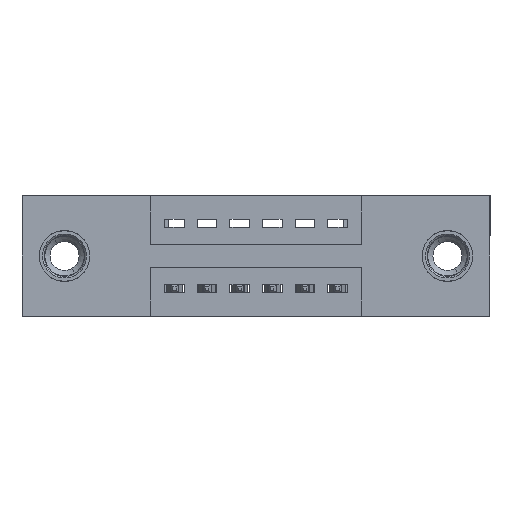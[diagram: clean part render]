
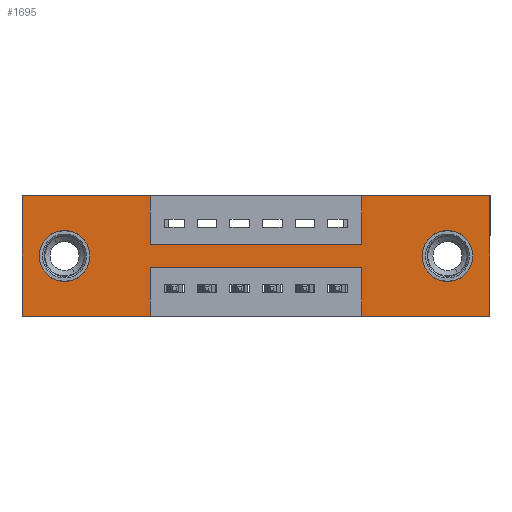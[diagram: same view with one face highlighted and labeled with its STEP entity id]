
A CAD part, front view. The second image highlights one B-rep face of the part: STEP entity #1695.
In plain terms, the highlighted planar face has unit normal (0, -1, 0).
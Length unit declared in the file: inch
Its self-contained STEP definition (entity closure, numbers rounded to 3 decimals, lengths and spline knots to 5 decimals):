
#74 = VECTOR ( 'NONE', #6606, 39.37008 ) ;
#309 = AXIS2_PLACEMENT_3D ( 'NONE', #6542, #10901, #5456 ) ;
#311 = FACE_OUTER_BOUND ( 'NONE', #3022, .T. ) ;
#397 = LINE ( 'NONE', #5510, #74 ) ;
#507 = VERTEX_POINT ( 'NONE', #11267 ) ;
#518 = CARTESIAN_POINT ( 'NONE',  ( 1.0425, 0., -0.22 ) ) ;
#690 = CIRCLE ( 'NONE', #8399, 0.078 ) ;
#788 = VERTEX_POINT ( 'NONE', #11175 ) ;
#956 = VERTEX_POINT ( 'NONE', #5908 ) ;
#1000 = VERTEX_POINT ( 'NONE', #10534 ) ;
#1104 = AXIS2_PLACEMENT_3D ( 'NONE', #5994, #8151, #4894 ) ;
#1392 = EDGE_CURVE ( 'NONE', #956, #8278, #1868, .T. ) ;
#1492 = ORIENTED_EDGE ( 'NONE', *, *, #8976, .F. ) ;
#1536 = ORIENTED_EDGE ( 'NONE', *, *, #10823, .T. ) ;
#1582 = CARTESIAN_POINT ( 'NONE',  ( 0., 0., -0.37 ) ) ;
#1606 = LINE ( 'NONE', #8634, #13543 ) ;
#1695 = ADVANCED_FACE ( 'NONE', ( #12281, #9045, #311 ), #2834, .T. ) ;
#1771 = DIRECTION ( 'NONE',  ( -1., 0., 0. ) ) ;
#1868 = CIRCLE ( 'NONE', #9289, 0.078 ) ;
#1903 = VERTEX_POINT ( 'NONE', #7016 ) ;
#1915 = CARTESIAN_POINT ( 'NONE',  ( 1.0425, 0., -0.37 ) ) ;
#1928 = ORIENTED_EDGE ( 'NONE', *, *, #3290, .F. ) ;
#2339 = VECTOR ( 'NONE', #7646, 39.37008 ) ;
#2377 = DIRECTION ( 'NONE',  ( 1., 0., 0. ) ) ;
#2423 = VERTEX_POINT ( 'NONE', #12396 ) ;
#2514 = EDGE_CURVE ( 'NONE', #3822, #8650, #5929, .T. ) ;
#2618 = ORIENTED_EDGE ( 'NONE', *, *, #8260, .F. ) ;
#2637 = ORIENTED_EDGE ( 'NONE', *, *, #5475, .F. ) ;
#2798 = AXIS2_PLACEMENT_3D ( 'NONE', #13715, #9388, #8246 ) ;
#2834 = PLANE ( 'NONE',  #2798 ) ;
#2943 = DIRECTION ( 'NONE',  ( 0., 0., 1. ) ) ;
#3022 = EDGE_LOOP ( 'NONE', ( #2618, #10832, #9074, #12781, #4828, #5292, #6846, #13736, #1928, #1492, #11619, #2637 ) ) ;
#3081 = CARTESIAN_POINT ( 'NONE',  ( 0.3925, 0., -0.15 ) ) ;
#3090 = LINE ( 'NONE', #3841, #5827 ) ;
#3159 = DIRECTION ( 'NONE',  ( 0., 0., 1. ) ) ;
#3215 = EDGE_CURVE ( 'NONE', #788, #1000, #3816, .T. ) ;
#3290 = EDGE_CURVE ( 'NONE', #1903, #788, #1606, .T. ) ;
#3531 = LINE ( 'NONE', #7357, #7301 ) ;
#3583 = VECTOR ( 'NONE', #1771, 39.37008 ) ;
#3816 = LINE ( 'NONE', #3081, #12546 ) ;
#3822 = VERTEX_POINT ( 'NONE', #10755 ) ;
#3833 = VECTOR ( 'NONE', #6990, 39.37008 ) ;
#3841 = CARTESIAN_POINT ( 'NONE',  ( 0., 0., -0.37 ) ) ;
#4026 = CARTESIAN_POINT ( 'NONE',  ( 1.305, 0., -0.107 ) ) ;
#4513 = DIRECTION ( 'NONE',  ( 0., 0., -1. ) ) ;
#4688 = CARTESIAN_POINT ( 'NONE',  ( 0., 0., 0. ) ) ;
#4800 = CARTESIAN_POINT ( 'NONE',  ( 0.3925, 0., -0.22 ) ) ;
#4828 = ORIENTED_EDGE ( 'NONE', *, *, #9532, .F. ) ;
#4894 = DIRECTION ( 'NONE',  ( 0., 0., -1. ) ) ;
#4933 = ORIENTED_EDGE ( 'NONE', *, *, #14075, .T. ) ;
#5292 = ORIENTED_EDGE ( 'NONE', *, *, #12111, .F. ) ;
#5301 = LINE ( 'NONE', #1582, #3583 ) ;
#5400 = CIRCLE ( 'NONE', #1104, 0.078 ) ;
#5426 = DIRECTION ( 'NONE',  ( 0., 0., 1. ) ) ;
#5456 = DIRECTION ( 'NONE',  ( 0., 0., 1. ) ) ;
#5467 = DIRECTION ( 'NONE',  ( 0., 1., 0. ) ) ;
#5475 = EDGE_CURVE ( 'NONE', #10353, #507, #5301, .T. ) ;
#5510 = CARTESIAN_POINT ( 'NONE',  ( 0., 0., 0. ) ) ;
#5827 = VECTOR ( 'NONE', #13760, 39.37008 ) ;
#5908 = CARTESIAN_POINT ( 'NONE',  ( 0.13, 0., -0.107 ) ) ;
#5929 = LINE ( 'NONE', #1915, #9528 ) ;
#5994 = CARTESIAN_POINT ( 'NONE',  ( 1.305, 0., -0.185 ) ) ;
#6279 = DIRECTION ( 'NONE',  ( 1., 0., 0. ) ) ;
#6542 = CARTESIAN_POINT ( 'NONE',  ( 0.13, 0., -0.185 ) ) ;
#6561 = CARTESIAN_POINT ( 'NONE',  ( 0.13, 0., -0.185 ) ) ;
#6584 = CARTESIAN_POINT ( 'NONE',  ( 0.3925, 0., -0.37 ) ) ;
#6606 = DIRECTION ( 'NONE',  ( 1., 0., 0. ) ) ;
#6846 = ORIENTED_EDGE ( 'NONE', *, *, #7122, .F. ) ;
#6886 = VERTEX_POINT ( 'NONE', #7288 ) ;
#6990 = DIRECTION ( 'NONE',  ( -1., 0., 0. ) ) ;
#7016 = CARTESIAN_POINT ( 'NONE',  ( 0.3925, 0., 0. ) ) ;
#7122 = EDGE_CURVE ( 'NONE', #1000, #12155, #3531, .T. ) ;
#7231 = EDGE_LOOP ( 'NONE', ( #8929, #4933 ) ) ;
#7288 = CARTESIAN_POINT ( 'NONE',  ( 1.435, 0., 0. ) ) ;
#7301 = VECTOR ( 'NONE', #3159, 39.37008 ) ;
#7357 = CARTESIAN_POINT ( 'NONE',  ( 1.0425, 0., 0. ) ) ;
#7638 = LINE ( 'NONE', #6584, #2339 ) ;
#7646 = DIRECTION ( 'NONE',  ( 0., 0., -1. ) ) ;
#7792 = LINE ( 'NONE', #8923, #13579 ) ;
#7817 = CARTESIAN_POINT ( 'NONE',  ( 0.3925, 0., -0.37 ) ) ;
#7849 = VERTEX_POINT ( 'NONE', #11430 ) ;
#7851 = CARTESIAN_POINT ( 'NONE',  ( 1.305, 0., -0.185 ) ) ;
#7939 = DIRECTION ( 'NONE',  ( 0., 1., 0. ) ) ;
#7961 = EDGE_CURVE ( 'NONE', #9775, #2423, #5400, .T. ) ;
#8151 = DIRECTION ( 'NONE',  ( 0., 1., 0. ) ) ;
#8246 = DIRECTION ( 'NONE',  ( 0., 0., -1. ) ) ;
#8260 = EDGE_CURVE ( 'NONE', #13501, #10353, #7638, .T. ) ;
#8278 = VERTEX_POINT ( 'NONE', #10941 ) ;
#8399 = AXIS2_PLACEMENT_3D ( 'NONE', #7851, #7939, #4513 ) ;
#8630 = LINE ( 'NONE', #11278, #12056 ) ;
#8634 = CARTESIAN_POINT ( 'NONE',  ( 0.3925, 0., 0. ) ) ;
#8650 = VERTEX_POINT ( 'NONE', #518 ) ;
#8923 = CARTESIAN_POINT ( 'NONE',  ( 0., 0., 0. ) ) ;
#8929 = ORIENTED_EDGE ( 'NONE', *, *, #7961, .T. ) ;
#8959 = ORIENTED_EDGE ( 'NONE', *, *, #1392, .T. ) ;
#8976 = EDGE_CURVE ( 'NONE', #7849, #1903, #7792, .T. ) ;
#9045 = FACE_BOUND ( 'NONE', #11641, .T. ) ;
#9054 = DIRECTION ( 'NONE',  ( 0., 0., -1. ) ) ;
#9074 = ORIENTED_EDGE ( 'NONE', *, *, #2514, .F. ) ;
#9289 = AXIS2_PLACEMENT_3D ( 'NONE', #6561, #5467, #5426 ) ;
#9388 = DIRECTION ( 'NONE',  ( 0., -1., 0. ) ) ;
#9508 = EDGE_CURVE ( 'NONE', #8650, #13501, #11539, .T. ) ;
#9528 = VECTOR ( 'NONE', #9552, 39.37008 ) ;
#9532 = EDGE_CURVE ( 'NONE', #6886, #10558, #8630, .T. ) ;
#9552 = DIRECTION ( 'NONE',  ( 0., 0., 1. ) ) ;
#9775 = VERTEX_POINT ( 'NONE', #4026 ) ;
#9892 = LINE ( 'NONE', #4688, #12656 ) ;
#10007 = CIRCLE ( 'NONE', #309, 0.078 ) ;
#10031 = EDGE_CURVE ( 'NONE', #507, #7849, #9892, .T. ) ;
#10353 = VERTEX_POINT ( 'NONE', #7817 ) ;
#10534 = CARTESIAN_POINT ( 'NONE',  ( 1.0425, 0., -0.15 ) ) ;
#10558 = VERTEX_POINT ( 'NONE', #12588 ) ;
#10755 = CARTESIAN_POINT ( 'NONE',  ( 1.0425, 0., -0.37 ) ) ;
#10823 = EDGE_CURVE ( 'NONE', #8278, #956, #10007, .T. ) ;
#10832 = ORIENTED_EDGE ( 'NONE', *, *, #9508, .F. ) ;
#10901 = DIRECTION ( 'NONE',  ( 0., 1., 0. ) ) ;
#10941 = CARTESIAN_POINT ( 'NONE',  ( 0.13, 0., -0.263 ) ) ;
#11155 = CARTESIAN_POINT ( 'NONE',  ( 1.0425, 0., 0. ) ) ;
#11175 = CARTESIAN_POINT ( 'NONE',  ( 0.3925, 0., -0.15 ) ) ;
#11267 = CARTESIAN_POINT ( 'NONE',  ( 0., 0., -0.37 ) ) ;
#11278 = CARTESIAN_POINT ( 'NONE',  ( 1.435, 0., 0. ) ) ;
#11423 = CARTESIAN_POINT ( 'NONE',  ( 0.3925, 0., -0.22 ) ) ;
#11430 = CARTESIAN_POINT ( 'NONE',  ( 0., 0., 0. ) ) ;
#11539 = LINE ( 'NONE', #11423, #3833 ) ;
#11619 = ORIENTED_EDGE ( 'NONE', *, *, #10031, .F. ) ;
#11641 = EDGE_LOOP ( 'NONE', ( #8959, #1536 ) ) ;
#12056 = VECTOR ( 'NONE', #9054, 39.37008 ) ;
#12068 = DIRECTION ( 'NONE',  ( 0., 0., -1. ) ) ;
#12111 = EDGE_CURVE ( 'NONE', #12155, #6886, #397, .T. ) ;
#12155 = VERTEX_POINT ( 'NONE', #11155 ) ;
#12281 = FACE_BOUND ( 'NONE', #7231, .T. ) ;
#12396 = CARTESIAN_POINT ( 'NONE',  ( 1.305, 0., -0.263 ) ) ;
#12546 = VECTOR ( 'NONE', #6279, 39.37008 ) ;
#12588 = CARTESIAN_POINT ( 'NONE',  ( 1.435, 0., -0.37 ) ) ;
#12656 = VECTOR ( 'NONE', #2943, 39.37008 ) ;
#12781 = ORIENTED_EDGE ( 'NONE', *, *, #13671, .F. ) ;
#13501 = VERTEX_POINT ( 'NONE', #4800 ) ;
#13543 = VECTOR ( 'NONE', #12068, 39.37008 ) ;
#13579 = VECTOR ( 'NONE', #2377, 39.37008 ) ;
#13671 = EDGE_CURVE ( 'NONE', #10558, #3822, #3090, .T. ) ;
#13715 = CARTESIAN_POINT ( 'NONE',  ( 0., 0., -0.37 ) ) ;
#13736 = ORIENTED_EDGE ( 'NONE', *, *, #3215, .F. ) ;
#13760 = DIRECTION ( 'NONE',  ( -1., 0., 0. ) ) ;
#14075 = EDGE_CURVE ( 'NONE', #2423, #9775, #690, .T. ) ;
